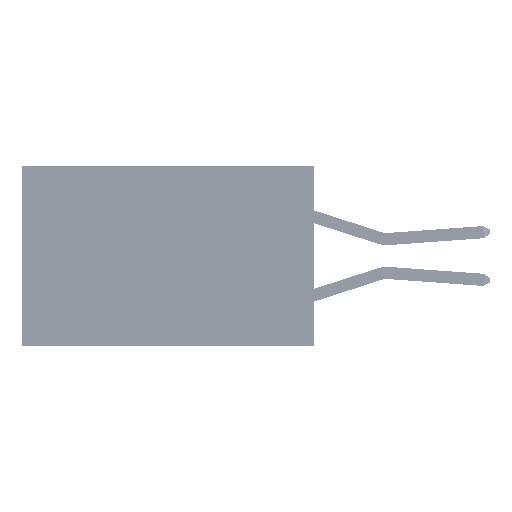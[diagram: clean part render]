
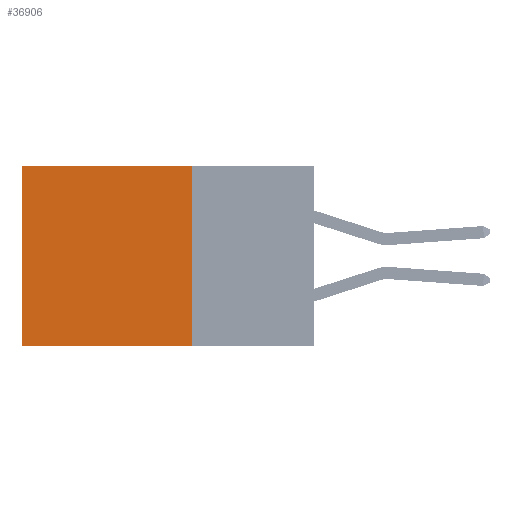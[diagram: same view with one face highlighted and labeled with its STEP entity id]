
A CAD part, left-side view. The second image highlights one B-rep face of the part: STEP entity #36906.
In plain terms, the highlighted planar face has unit normal (-1, 0, 0).
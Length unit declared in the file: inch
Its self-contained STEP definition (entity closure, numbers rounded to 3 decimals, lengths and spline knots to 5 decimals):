
#1035 = CARTESIAN_POINT ( 'NONE',  ( 0.2875, 0.6, 0. ) ) ;
#3153 = VECTOR ( 'NONE', #31389, 39.37008 ) ;
#4407 = VECTOR ( 'NONE', #13140, 39.37008 ) ;
#6084 = CARTESIAN_POINT ( 'NONE',  ( 0.2875, 0.25, -0.37 ) ) ;
#6920 = EDGE_CURVE ( 'NONE', #24853, #31386, #11565, .T. ) ;
#7388 = AXIS2_PLACEMENT_3D ( 'NONE', #24138, #19898, #41957 ) ;
#7931 = DIRECTION ( 'NONE',  ( 0., 0., -1. ) ) ;
#10417 = FACE_OUTER_BOUND ( 'NONE', #34926, .T. ) ;
#11565 = LINE ( 'NONE', #1035, #43118 ) ;
#12481 = LINE ( 'NONE', #17644, #23211 ) ;
#13140 = DIRECTION ( 'NONE',  ( 0., 1., 0. ) ) ;
#13933 = LINE ( 'NONE', #6084, #4407 ) ;
#14880 = EDGE_CURVE ( 'NONE', #18816, #22186, #12481, .T. ) ;
#17644 = CARTESIAN_POINT ( 'NONE',  ( 0.2875, 0.25, 0. ) ) ;
#18816 = VERTEX_POINT ( 'NONE', #19452 ) ;
#19452 = CARTESIAN_POINT ( 'NONE',  ( 0.2875, 0.25, 0. ) ) ;
#19898 = DIRECTION ( 'NONE',  ( 1., 0., 0. ) ) ;
#20047 = CARTESIAN_POINT ( 'NONE',  ( 0.2875, 0.25, 0. ) ) ;
#20791 = ORIENTED_EDGE ( 'NONE', *, *, #14880, .F. ) ;
#22186 = VERTEX_POINT ( 'NONE', #33063 ) ;
#23211 = VECTOR ( 'NONE', #24870, 39.37008 ) ;
#24138 = CARTESIAN_POINT ( 'NONE',  ( 0.2875, 0.25, 0. ) ) ;
#24853 = VERTEX_POINT ( 'NONE', #26386 ) ;
#24870 = DIRECTION ( 'NONE',  ( 0., 0., -1. ) ) ;
#26300 = ORIENTED_EDGE ( 'NONE', *, *, #6920, .T. ) ;
#26386 = CARTESIAN_POINT ( 'NONE',  ( 0.2875, 0.6, 0. ) ) ;
#28517 = CARTESIAN_POINT ( 'NONE',  ( 0.2875, 0.6, -0.37 ) ) ;
#31386 = VERTEX_POINT ( 'NONE', #28517 ) ;
#31389 = DIRECTION ( 'NONE',  ( 0., 1., 0. ) ) ;
#32357 = LINE ( 'NONE', #20047, #3153 ) ;
#33063 = CARTESIAN_POINT ( 'NONE',  ( 0.2875, 0.25, -0.37 ) ) ;
#33414 = ORIENTED_EDGE ( 'NONE', *, *, #37947, .F. ) ;
#34926 = EDGE_LOOP ( 'NONE', ( #26300, #33414, #20791, #45954 ) ) ;
#36882 = EDGE_CURVE ( 'NONE', #18816, #24853, #32357, .T. ) ;
#36906 = ADVANCED_FACE ( 'NONE', ( #10417 ), #38307, .F. ) ;
#37947 = EDGE_CURVE ( 'NONE', #22186, #31386, #13933, .T. ) ;
#38307 = PLANE ( 'NONE',  #7388 ) ;
#41957 = DIRECTION ( 'NONE',  ( 0., 0., -1. ) ) ;
#43118 = VECTOR ( 'NONE', #7931, 39.37008 ) ;
#45954 = ORIENTED_EDGE ( 'NONE', *, *, #36882, .T. ) ;
